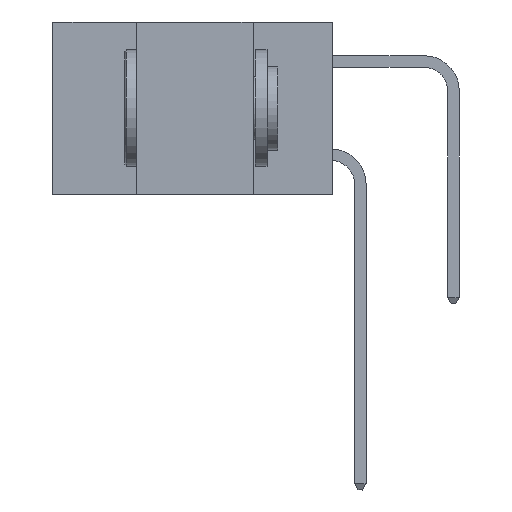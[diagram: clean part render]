
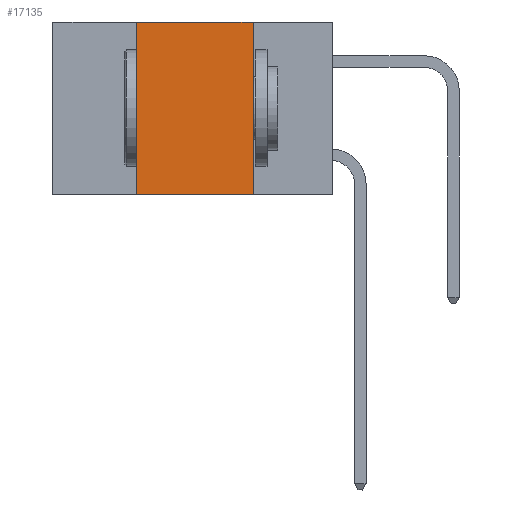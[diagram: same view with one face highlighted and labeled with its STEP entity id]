
A CAD part, left-side view. The second image highlights one B-rep face of the part: STEP entity #17135.
In plain terms, the highlighted planar face has unit normal (-1, 0, 0).
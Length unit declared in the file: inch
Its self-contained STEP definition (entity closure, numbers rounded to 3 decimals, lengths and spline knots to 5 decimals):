
#1486 = CARTESIAN_POINT ( 'NONE',  ( 0., 0.17, 0. ) ) ;
#1735 = DIRECTION ( 'NONE',  ( 0., 0., -1. ) ) ;
#1762 = VECTOR ( 'NONE', #10918, 39.37008 ) ;
#1792 = CARTESIAN_POINT ( 'NONE',  ( 0., 0.42, 0. ) ) ;
#2262 = CARTESIAN_POINT ( 'NONE',  ( 0., 0.6, 0. ) ) ;
#2767 = EDGE_LOOP ( 'NONE', ( #6266, #5642, #7339, #3719 ) ) ;
#2920 = CARTESIAN_POINT ( 'NONE',  ( 0., 0.6, -0.37 ) ) ;
#3433 = DIRECTION ( 'NONE',  ( 0., 0., 1. ) ) ;
#3719 = ORIENTED_EDGE ( 'NONE', *, *, #12740, .T. ) ;
#3900 = DIRECTION ( 'NONE',  ( 1., 0., 0. ) ) ;
#5642 = ORIENTED_EDGE ( 'NONE', *, *, #18653, .F. ) ;
#6050 = LINE ( 'NONE', #2920, #1762 ) ;
#6266 = ORIENTED_EDGE ( 'NONE', *, *, #18876, .F. ) ;
#6284 = AXIS2_PLACEMENT_3D ( 'NONE', #2262, #3900, #14924 ) ;
#7105 = LINE ( 'NONE', #1792, #11352 ) ;
#7339 = ORIENTED_EDGE ( 'NONE', *, *, #14783, .F. ) ;
#7928 = CARTESIAN_POINT ( 'NONE',  ( 0., 0.42, -0.37 ) ) ;
#8138 = CARTESIAN_POINT ( 'NONE',  ( 0., 0.17, 0. ) ) ;
#9495 = CARTESIAN_POINT ( 'NONE',  ( 0., 0.42, 0. ) ) ;
#9969 = VERTEX_POINT ( 'NONE', #7928 ) ;
#10702 = VECTOR ( 'NONE', #15282, 39.37008 ) ;
#10918 = DIRECTION ( 'NONE',  ( 0., -1., 0. ) ) ;
#10925 = VECTOR ( 'NONE', #1735, 39.37008 ) ;
#11270 = VERTEX_POINT ( 'NONE', #9495 ) ;
#11352 = VECTOR ( 'NONE', #3433, 39.37008 ) ;
#11858 = PLANE ( 'NONE',  #6284 ) ;
#12160 = VERTEX_POINT ( 'NONE', #1486 ) ;
#12740 = EDGE_CURVE ( 'NONE', #9969, #15833, #6050, .T. ) ;
#14759 = LINE ( 'NONE', #16826, #10702 ) ;
#14783 = EDGE_CURVE ( 'NONE', #9969, #11270, #7105, .T. ) ;
#14924 = DIRECTION ( 'NONE',  ( 0., 0., -1. ) ) ;
#15109 = CARTESIAN_POINT ( 'NONE',  ( 0., 0.17, -0.37 ) ) ;
#15282 = DIRECTION ( 'NONE',  ( 0., -1., 0. ) ) ;
#15833 = VERTEX_POINT ( 'NONE', #15109 ) ;
#16826 = CARTESIAN_POINT ( 'NONE',  ( 0., 0.6, 0. ) ) ;
#17135 = ADVANCED_FACE ( 'NONE', ( #19124 ), #11858, .F. ) ;
#18653 = EDGE_CURVE ( 'NONE', #11270, #12160, #14759, .T. ) ;
#18876 = EDGE_CURVE ( 'NONE', #12160, #15833, #19051, .T. ) ;
#19051 = LINE ( 'NONE', #8138, #10925 ) ;
#19124 = FACE_OUTER_BOUND ( 'NONE', #2767, .T. ) ;
